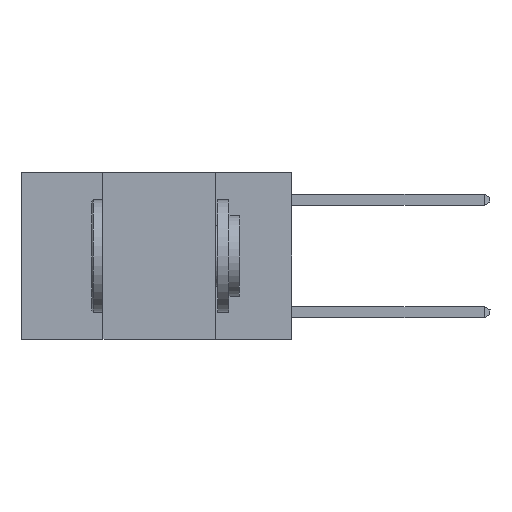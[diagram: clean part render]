
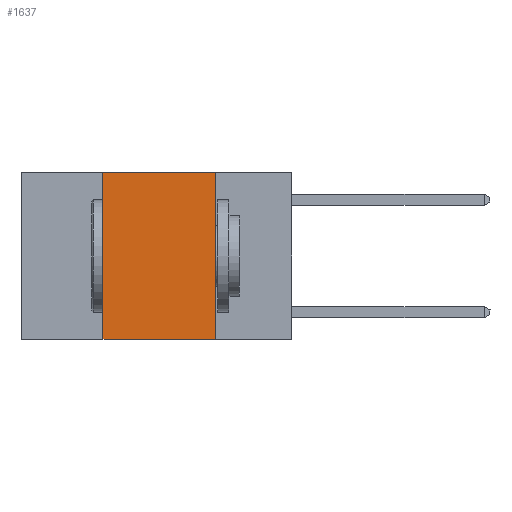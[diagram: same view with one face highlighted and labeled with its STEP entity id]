
A CAD part, left-side view. The second image highlights one B-rep face of the part: STEP entity #1637.
In plain terms, the highlighted planar face has unit normal (-1, 0, 0).
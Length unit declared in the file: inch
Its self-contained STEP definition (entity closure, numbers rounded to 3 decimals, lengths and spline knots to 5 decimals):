
#299 = DIRECTION ( 'NONE',  ( 1., 0., 0. ) ) ;
#468 = EDGE_CURVE ( 'NONE', #20970, #17564, #4901, .T. ) ;
#904 = VECTOR ( 'NONE', #9662, 39.37008 ) ;
#1637 = ADVANCED_FACE ( 'NONE', ( #18600 ), #26527, .F. ) ;
#1658 = VERTEX_POINT ( 'NONE', #22532 ) ;
#2108 = CARTESIAN_POINT ( 'NONE',  ( 0., 0.42, 0. ) ) ;
#3214 = CARTESIAN_POINT ( 'NONE',  ( 0., 0.17, 0. ) ) ;
#3492 = VECTOR ( 'NONE', #28099, 39.37008 ) ;
#4901 = LINE ( 'NONE', #8650, #15983 ) ;
#6835 = LINE ( 'NONE', #20639, #904 ) ;
#7416 = DIRECTION ( 'NONE',  ( 0., -1., 0. ) ) ;
#7531 = CARTESIAN_POINT ( 'NONE',  ( 0., 0.42, 0. ) ) ;
#7619 = CARTESIAN_POINT ( 'NONE',  ( 0., 0.17, -0.37 ) ) ;
#8082 = VECTOR ( 'NONE', #20840, 39.37008 ) ;
#8650 = CARTESIAN_POINT ( 'NONE',  ( 0., 0.6, 0. ) ) ;
#9662 = DIRECTION ( 'NONE',  ( 0., -1., 0. ) ) ;
#14570 = VERTEX_POINT ( 'NONE', #7619 ) ;
#15419 = LINE ( 'NONE', #3214, #8082 ) ;
#15935 = DIRECTION ( 'NONE',  ( 0., 0., -1. ) ) ;
#15983 = VECTOR ( 'NONE', #7416, 39.37008 ) ;
#17564 = VERTEX_POINT ( 'NONE', #23724 ) ;
#18075 = EDGE_CURVE ( 'NONE', #17564, #14570, #15419, .T. ) ;
#18600 = FACE_OUTER_BOUND ( 'NONE', #22531, .T. ) ;
#20565 = AXIS2_PLACEMENT_3D ( 'NONE', #22335, #299, #15935 ) ;
#20596 = EDGE_CURVE ( 'NONE', #1658, #20970, #21056, .T. ) ;
#20639 = CARTESIAN_POINT ( 'NONE',  ( 0., 0.6, -0.37 ) ) ;
#20840 = DIRECTION ( 'NONE',  ( 0., 0., -1. ) ) ;
#20970 = VERTEX_POINT ( 'NONE', #7531 ) ;
#21056 = LINE ( 'NONE', #2108, #3492 ) ;
#22335 = CARTESIAN_POINT ( 'NONE',  ( 0., 0.6, 0. ) ) ;
#22531 = EDGE_LOOP ( 'NONE', ( #25855, #25897, #26087, #26094 ) ) ;
#22532 = CARTESIAN_POINT ( 'NONE',  ( 0., 0.42, -0.37 ) ) ;
#23724 = CARTESIAN_POINT ( 'NONE',  ( 0., 0.17, 0. ) ) ;
#25855 = ORIENTED_EDGE ( 'NONE', *, *, #18075, .F. ) ;
#25897 = ORIENTED_EDGE ( 'NONE', *, *, #468, .F. ) ;
#26087 = ORIENTED_EDGE ( 'NONE', *, *, #20596, .F. ) ;
#26094 = ORIENTED_EDGE ( 'NONE', *, *, #28091, .T. ) ;
#26527 = PLANE ( 'NONE',  #20565 ) ;
#28091 = EDGE_CURVE ( 'NONE', #1658, #14570, #6835, .T. ) ;
#28099 = DIRECTION ( 'NONE',  ( 0., 0., 1. ) ) ;
